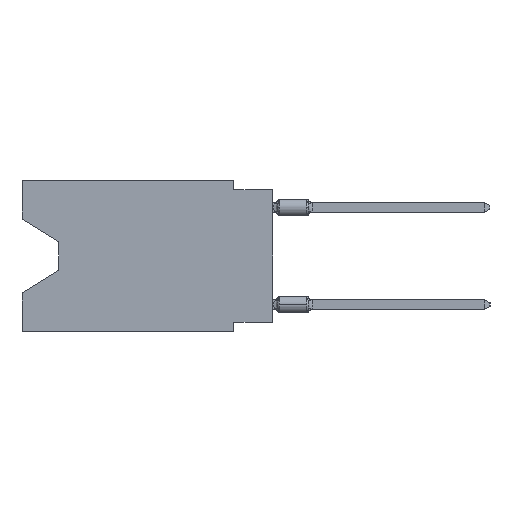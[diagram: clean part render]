
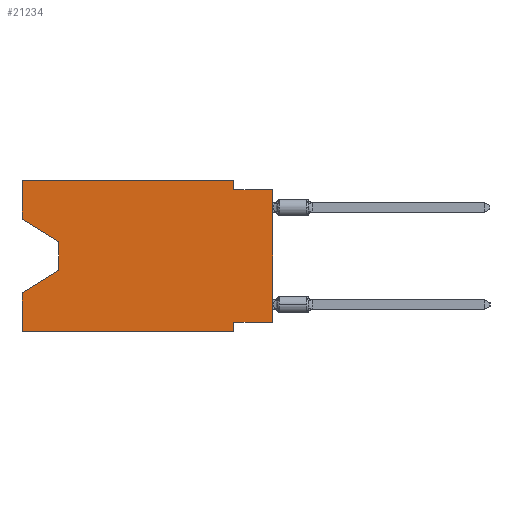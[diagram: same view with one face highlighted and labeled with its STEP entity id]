
A CAD part, left-side view. The second image highlights one B-rep face of the part: STEP entity #21234.
In plain terms, the highlighted planar face has unit normal (-1, 0, 0).
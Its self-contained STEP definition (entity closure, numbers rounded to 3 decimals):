
#49 = LINE ( 'NONE', #35320, #21130 ) ;
#738 = CARTESIAN_POINT ( 'NONE',  ( 0., 13.97, -5.893 ) ) ;
#1021 = EDGE_CURVE ( 'NONE', #19590, #9338, #10526, .T. ) ;
#1323 = LINE ( 'NONE', #31388, #4609 ) ;
#1366 = CARTESIAN_POINT ( 'NONE',  ( 0., 2.54, -9.271 ) ) ;
#1444 = VECTOR ( 'NONE', #30582, 1000. ) ;
#2000 = VERTEX_POINT ( 'NONE', #19703 ) ;
#2210 = ORIENTED_EDGE ( 'NONE', *, *, #2331, .F. ) ;
#2245 = VERTEX_POINT ( 'NONE', #13009 ) ;
#2331 = EDGE_CURVE ( 'NONE', #32003, #8171, #16812, .T. ) ;
#3175 = VERTEX_POINT ( 'NONE', #22420 ) ;
#3239 = CARTESIAN_POINT ( 'NONE',  ( 0., 16.383, -9.906 ) ) ;
#3464 = CARTESIAN_POINT ( 'NONE',  ( 0., 2.54, -0.635 ) ) ;
#4388 = CARTESIAN_POINT ( 'NONE',  ( 0., 0., -9.271 ) ) ;
#4609 = VECTOR ( 'NONE', #6867, 1000. ) ;
#4628 = VERTEX_POINT ( 'NONE', #27657 ) ;
#5184 = DIRECTION ( 'NONE',  ( 0., 0., -1. ) ) ;
#5301 = CARTESIAN_POINT ( 'NONE',  ( 0., 16.383, -2.546 ) ) ;
#5393 = EDGE_CURVE ( 'NONE', #13689, #9338, #30066, .T. ) ;
#5398 = LINE ( 'NONE', #7716, #13184 ) ;
#5623 = VECTOR ( 'NONE', #10901, 1000. ) ;
#5883 = EDGE_CURVE ( 'NONE', #9546, #13405, #23300, .T. ) ;
#6224 = CARTESIAN_POINT ( 'NONE',  ( 0., 16.383, -2.546 ) ) ;
#6429 = DIRECTION ( 'NONE',  ( 0., 0., -1. ) ) ;
#6840 = EDGE_CURVE ( 'NONE', #2245, #2000, #49, .T. ) ;
#6867 = DIRECTION ( 'NONE',  ( 0., -1., 0. ) ) ;
#7716 = CARTESIAN_POINT ( 'NONE',  ( 0., 2.54, -9.906 ) ) ;
#8171 = VERTEX_POINT ( 'NONE', #1366 ) ;
#8850 = ORIENTED_EDGE ( 'NONE', *, *, #24282, .T. ) ;
#8878 = CARTESIAN_POINT ( 'NONE',  ( 0., 0., -0.635 ) ) ;
#9338 = VERTEX_POINT ( 'NONE', #23018 ) ;
#9546 = VERTEX_POINT ( 'NONE', #3464 ) ;
#9593 = CARTESIAN_POINT ( 'NONE',  ( 0., 0., 0. ) ) ;
#10010 = LINE ( 'NONE', #21318, #13209 ) ;
#10202 = VECTOR ( 'NONE', #20636, 1000. ) ;
#10526 = LINE ( 'NONE', #21618, #32501 ) ;
#10901 = DIRECTION ( 'NONE',  ( 0., 0., 1. ) ) ;
#11106 = ORIENTED_EDGE ( 'NONE', *, *, #30575, .F. ) ;
#11123 = CARTESIAN_POINT ( 'NONE',  ( 0., 16.383, 0. ) ) ;
#11315 = DIRECTION ( 'NONE',  ( 0., -1., 0. ) ) ;
#11449 = VECTOR ( 'NONE', #18721, 1000. ) ;
#13009 = CARTESIAN_POINT ( 'NONE',  ( 0., 16.383, 0. ) ) ;
#13184 = VECTOR ( 'NONE', #35127, 1000. ) ;
#13209 = VECTOR ( 'NONE', #5184, 1000. ) ;
#13267 = PLANE ( 'NONE',  #18895 ) ;
#13405 = VERTEX_POINT ( 'NONE', #20323 ) ;
#13689 = VERTEX_POINT ( 'NONE', #3239 ) ;
#14471 = VECTOR ( 'NONE', #31272, 1000. ) ;
#15596 = DIRECTION ( 'NONE',  ( 0., 0., -1. ) ) ;
#15819 = ORIENTED_EDGE ( 'NONE', *, *, #33020, .F. ) ;
#16514 = EDGE_CURVE ( 'NONE', #13689, #3175, #1323, .T. ) ;
#16812 = LINE ( 'NONE', #31090, #1444 ) ;
#17816 = ORIENTED_EDGE ( 'NONE', *, *, #5393, .F. ) ;
#18631 = CARTESIAN_POINT ( 'NONE',  ( 0., 16.383, 0. ) ) ;
#18721 = DIRECTION ( 'NONE',  ( 0., -0.855, -0.519 ) ) ;
#18895 = AXIS2_PLACEMENT_3D ( 'NONE', #18631, #34932, #15596 ) ;
#18931 = EDGE_CURVE ( 'NONE', #32003, #13405, #20367, .T. ) ;
#19300 = EDGE_LOOP ( 'NONE', ( #8850, #30948, #32342, #17816, #26965, #32299, #2210, #21581, #19905, #11106, #32543, #15819 ) ) ;
#19590 = VERTEX_POINT ( 'NONE', #738 ) ;
#19703 = CARTESIAN_POINT ( 'NONE',  ( 0., 2.54, 0. ) ) ;
#19905 = ORIENTED_EDGE ( 'NONE', *, *, #5883, .F. ) ;
#20040 = LINE ( 'NONE', #30968, #26259 ) ;
#20291 = EDGE_CURVE ( 'NONE', #4628, #19590, #20040, .T. ) ;
#20323 = CARTESIAN_POINT ( 'NONE',  ( 0., 0., -0.635 ) ) ;
#20367 = LINE ( 'NONE', #9593, #14471 ) ;
#20636 = DIRECTION ( 'NONE',  ( 0., -1., 0. ) ) ;
#21130 = VECTOR ( 'NONE', #11315, 1000. ) ;
#21234 = ADVANCED_FACE ( 'NONE', ( #32403 ), #13267, .F. ) ;
#21318 = CARTESIAN_POINT ( 'NONE',  ( 0., 2.54, 0. ) ) ;
#21581 = ORIENTED_EDGE ( 'NONE', *, *, #18931, .T. ) ;
#21618 = CARTESIAN_POINT ( 'NONE',  ( 0., 13.97, -5.893 ) ) ;
#21643 = CARTESIAN_POINT ( 'NONE',  ( 0., 16.383, 0. ) ) ;
#22054 = DIRECTION ( 'NONE',  ( 0., 0., 1. ) ) ;
#22420 = CARTESIAN_POINT ( 'NONE',  ( 0., 2.54, -9.906 ) ) ;
#23018 = CARTESIAN_POINT ( 'NONE',  ( 0., 16.383, -7.36 ) ) ;
#23300 = LINE ( 'NONE', #8878, #10202 ) ;
#24282 = EDGE_CURVE ( 'NONE', #34701, #4628, #32494, .T. ) ;
#26259 = VECTOR ( 'NONE', #6429, 1000. ) ;
#26378 = EDGE_CURVE ( 'NONE', #8171, #3175, #5398, .T. ) ;
#26965 = ORIENTED_EDGE ( 'NONE', *, *, #16514, .T. ) ;
#27009 = DIRECTION ( 'NONE',  ( 0., 0.855, -0.519 ) ) ;
#27657 = CARTESIAN_POINT ( 'NONE',  ( 0., 13.97, -4.013 ) ) ;
#29942 = VECTOR ( 'NONE', #22054, 1000. ) ;
#30066 = LINE ( 'NONE', #21643, #5623 ) ;
#30472 = LINE ( 'NONE', #11123, #29942 ) ;
#30575 = EDGE_CURVE ( 'NONE', #2000, #9546, #10010, .T. ) ;
#30582 = DIRECTION ( 'NONE',  ( 0., 1., 0. ) ) ;
#30948 = ORIENTED_EDGE ( 'NONE', *, *, #20291, .T. ) ;
#30968 = CARTESIAN_POINT ( 'NONE',  ( 0., 13.97, -4.013 ) ) ;
#31090 = CARTESIAN_POINT ( 'NONE',  ( 0., 0., -9.271 ) ) ;
#31272 = DIRECTION ( 'NONE',  ( 0., 0., 1. ) ) ;
#31388 = CARTESIAN_POINT ( 'NONE',  ( 0., 16.383, -9.906 ) ) ;
#32003 = VERTEX_POINT ( 'NONE', #4388 ) ;
#32299 = ORIENTED_EDGE ( 'NONE', *, *, #26378, .F. ) ;
#32342 = ORIENTED_EDGE ( 'NONE', *, *, #1021, .T. ) ;
#32403 = FACE_OUTER_BOUND ( 'NONE', #19300, .T. ) ;
#32494 = LINE ( 'NONE', #5301, #11449 ) ;
#32501 = VECTOR ( 'NONE', #27009, 1000. ) ;
#32543 = ORIENTED_EDGE ( 'NONE', *, *, #6840, .F. ) ;
#33020 = EDGE_CURVE ( 'NONE', #34701, #2245, #30472, .T. ) ;
#34701 = VERTEX_POINT ( 'NONE', #6224 ) ;
#34932 = DIRECTION ( 'NONE',  ( 1., 0., 0. ) ) ;
#35127 = DIRECTION ( 'NONE',  ( 0., 0., -1. ) ) ;
#35320 = CARTESIAN_POINT ( 'NONE',  ( 0., 16.383, 0. ) ) ;
